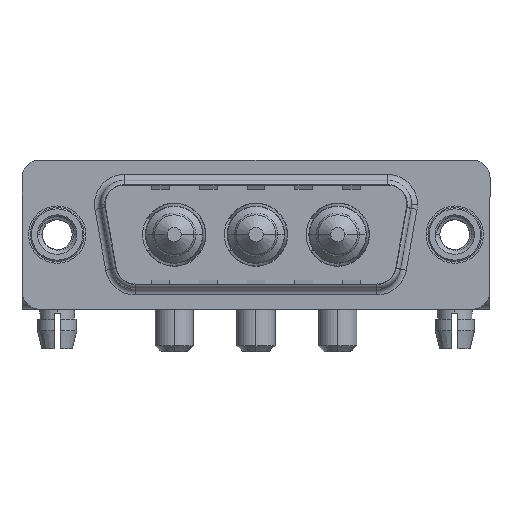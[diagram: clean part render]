
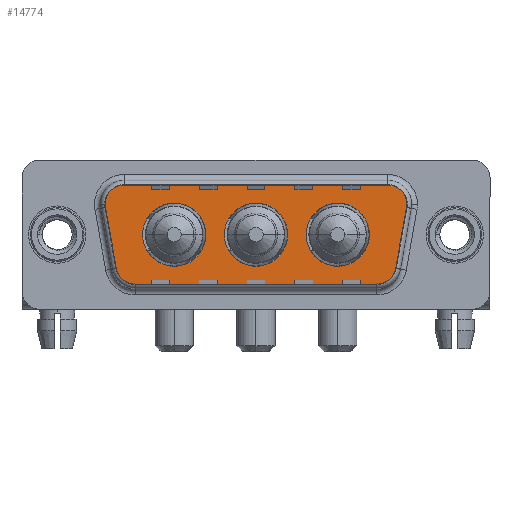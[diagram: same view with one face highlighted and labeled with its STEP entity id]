
A CAD part, top view. The second image highlights one B-rep face of the part: STEP entity #14774.
In plain terms, the highlighted planar face has unit normal (0, 0, 1).
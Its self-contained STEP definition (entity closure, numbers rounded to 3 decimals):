
#85 = AXIS2_PLACEMENT_3D ( 'NONE', #7280, #6156, #977 ) ;
#623 = DIRECTION ( 'NONE',  ( 0., 0., 1. ) ) ;
#839 = LINE ( 'NONE', #14089, #12455 ) ;
#970 = DIRECTION ( 'NONE',  ( 0., 0., 1. ) ) ;
#977 = DIRECTION ( 'NONE',  ( 1., 0., 0. ) ) ;
#1140 = CARTESIAN_POINT ( 'NONE',  ( 6.434, -4.9, 0. ) ) ;
#1514 = ORIENTED_EDGE ( 'NONE', *, *, #14882, .T. ) ;
#1573 = VERTEX_POINT ( 'NONE', #12220 ) ;
#1735 = CARTESIAN_POINT ( 'NONE',  ( 23.5, 0., 0. ) ) ;
#1796 = EDGE_CURVE ( 'NONE', #4521, #13586, #2761, .T. ) ;
#1833 = VERTEX_POINT ( 'NONE', #7849 ) ;
#2042 = DIRECTION ( 'NONE',  ( 0., 0., 1. ) ) ;
#2134 = DIRECTION ( 'NONE',  ( 0., 0., 1. ) ) ;
#2305 = CARTESIAN_POINT ( 'NONE',  ( 27.889, 4.9, 0. ) ) ;
#2618 = EDGE_CURVE ( 'NONE', #16424, #9800, #5568, .T. ) ;
#2658 = EDGE_CURVE ( 'NONE', #6936, #8131, #15450, .T. ) ;
#2761 = CIRCLE ( 'NONE', #7156, 2.65 ) ;
#3028 = DIRECTION ( 'NONE',  ( 0., 0., 1. ) ) ;
#3117 = VERTEX_POINT ( 'NONE', #4864 ) ;
#3252 = ORIENTED_EDGE ( 'NONE', *, *, #7204, .F. ) ;
#3288 = PLANE ( 'NONE',  #4502 ) ;
#3499 = DIRECTION ( 'NONE',  ( -1., 0., 0. ) ) ;
#3552 = AXIS2_PLACEMENT_3D ( 'NONE', #1735, #6993, #4160 ) ;
#3578 = EDGE_CURVE ( 'NONE', #7042, #1833, #839, .T. ) ;
#3691 = ORIENTED_EDGE ( 'NONE', *, *, #2618, .F. ) ;
#3872 = EDGE_LOOP ( 'NONE', ( #16402, #11729, #12885, #12441, #4454, #10476, #14609, #1514, #11324 ) ) ;
#3940 = ORIENTED_EDGE ( 'NONE', *, *, #1796, .F. ) ;
#3994 = AXIS2_PLACEMENT_3D ( 'NONE', #7100, #623, #4341 ) ;
#4160 = DIRECTION ( 'NONE',  ( 1., 0., 0. ) ) ;
#4191 = DIRECTION ( 'NONE',  ( 0., 0., 1. ) ) ;
#4214 = EDGE_CURVE ( 'NONE', #16069, #14965, #6508, .T. ) ;
#4341 = DIRECTION ( 'NONE',  ( 1., 0., 0. ) ) ;
#4454 = ORIENTED_EDGE ( 'NONE', *, *, #14383, .T. ) ;
#4468 = AXIS2_PLACEMENT_3D ( 'NONE', #15277, #2042, #3499 ) ;
#4502 = AXIS2_PLACEMENT_3D ( 'NONE', #6135, #11376, #7505 ) ;
#4521 = VERTEX_POINT ( 'NONE', #11869 ) ;
#4583 = ORIENTED_EDGE ( 'NONE', *, *, #13232, .F. ) ;
#4864 = CARTESIAN_POINT ( 'NONE',  ( 26.866, -4.9, 0. ) ) ;
#4932 = CARTESIAN_POINT ( 'NONE',  ( 6.434, -2.9, 0. ) ) ;
#4954 = CARTESIAN_POINT ( 'NONE',  ( 5.411, 4.9, 0. ) ) ;
#5054 = CARTESIAN_POINT ( 'NONE',  ( 29.889, 2.9, 0. ) ) ;
#5212 = DIRECTION ( 'NONE',  ( 0., 0., 1. ) ) ;
#5328 = VECTOR ( 'NONE', #10114, 1000. ) ;
#5332 = EDGE_CURVE ( 'NONE', #9641, #7042, #14146, .T. ) ;
#5568 = CIRCLE ( 'NONE', #6933, 2.65 ) ;
#5893 = AXIS2_PLACEMENT_3D ( 'NONE', #11986, #3028, #10776 ) ;
#6127 = DIRECTION ( 'NONE',  ( 0., 0., 1. ) ) ;
#6135 = CARTESIAN_POINT ( 'NONE',  ( 26.866, -2.9, 0. ) ) ;
#6156 = DIRECTION ( 'NONE',  ( 0., 0., 1. ) ) ;
#6275 = DIRECTION ( 'NONE',  ( 0.174, -0.985, 0. ) ) ;
#6508 = LINE ( 'NONE', #11746, #7497 ) ;
#6550 = DIRECTION ( 'NONE',  ( 1., 0., 0. ) ) ;
#6854 = VECTOR ( 'NONE', #7526, 1000. ) ;
#6855 = CARTESIAN_POINT ( 'NONE',  ( 28.836, -3.247, 0. ) ) ;
#6933 = AXIS2_PLACEMENT_3D ( 'NONE', #8158, #4191, #9444 ) ;
#6936 = VERTEX_POINT ( 'NONE', #5054 ) ;
#6993 = DIRECTION ( 'NONE',  ( 0., 0., 1. ) ) ;
#7033 = EDGE_CURVE ( 'NONE', #14965, #6936, #10509, .T. ) ;
#7042 = VERTEX_POINT ( 'NONE', #12782 ) ;
#7100 = CARTESIAN_POINT ( 'NONE',  ( 9.8, 0., 0. ) ) ;
#7156 = AXIS2_PLACEMENT_3D ( 'NONE', #7416, #6127, #6550 ) ;
#7166 = FACE_BOUND ( 'NONE', #11621, .T. ) ;
#7204 = EDGE_CURVE ( 'NONE', #9800, #16424, #10034, .T. ) ;
#7255 = DIRECTION ( 'NONE',  ( 0., 0., 1. ) ) ;
#7262 = AXIS2_PLACEMENT_3D ( 'NONE', #4932, #7255, #12490 ) ;
#7280 = CARTESIAN_POINT ( 'NONE',  ( 16.65, 0., 0. ) ) ;
#7416 = CARTESIAN_POINT ( 'NONE',  ( 16.65, 0., 0. ) ) ;
#7497 = VECTOR ( 'NONE', #15873, 1000. ) ;
#7505 = DIRECTION ( 'NONE',  ( 1., 0., 0. ) ) ;
#7526 = DIRECTION ( 'NONE',  ( 1., 0., 0. ) ) ;
#7819 = EDGE_LOOP ( 'NONE', ( #4583, #12108 ) ) ;
#7849 = CARTESIAN_POINT ( 'NONE',  ( 4.464, -3.247, 0. ) ) ;
#7879 = DIRECTION ( 'NONE',  ( 1., 0., 0. ) ) ;
#7903 = VERTEX_POINT ( 'NONE', #14605 ) ;
#8131 = VERTEX_POINT ( 'NONE', #2305 ) ;
#8158 = CARTESIAN_POINT ( 'NONE',  ( 9.8, 0., 0. ) ) ;
#8536 = EDGE_CURVE ( 'NONE', #13586, #4521, #14114, .T. ) ;
#8818 = LINE ( 'NONE', #14048, #6854 ) ;
#8842 = VERTEX_POINT ( 'NONE', #1140 ) ;
#8958 = EDGE_CURVE ( 'NONE', #1573, #7903, #16547, .T. ) ;
#9056 = CARTESIAN_POINT ( 'NONE',  ( 14., 0., 0. ) ) ;
#9444 = DIRECTION ( 'NONE',  ( 1., 0., 0. ) ) ;
#9641 = VERTEX_POINT ( 'NONE', #14588 ) ;
#9800 = VERTEX_POINT ( 'NONE', #13456 ) ;
#9999 = CIRCLE ( 'NONE', #14913, 2. ) ;
#10034 = CIRCLE ( 'NONE', #3994, 2.65 ) ;
#10114 = DIRECTION ( 'NONE',  ( -1., 0., 0. ) ) ;
#10476 = ORIENTED_EDGE ( 'NONE', *, *, #5332, .T. ) ;
#10509 = CIRCLE ( 'NONE', #11880, 2. ) ;
#10587 = ORIENTED_EDGE ( 'NONE', *, *, #8536, .F. ) ;
#10776 = DIRECTION ( 'NONE',  ( 1., 0., 0. ) ) ;
#11324 = ORIENTED_EDGE ( 'NONE', *, *, #12970, .T. ) ;
#11376 = DIRECTION ( 'NONE',  ( 0., 0., 1. ) ) ;
#11621 = EDGE_LOOP ( 'NONE', ( #3252, #3691 ) ) ;
#11680 = AXIS2_PLACEMENT_3D ( 'NONE', #16874, #970, #12917 ) ;
#11729 = ORIENTED_EDGE ( 'NONE', *, *, #4214, .T. ) ;
#11746 = CARTESIAN_POINT ( 'NONE',  ( 29.859, 2.553, 0. ) ) ;
#11869 = CARTESIAN_POINT ( 'NONE',  ( 19.3, 0., 0. ) ) ;
#11880 = AXIS2_PLACEMENT_3D ( 'NONE', #13903, #2134, #12689 ) ;
#11986 = CARTESIAN_POINT ( 'NONE',  ( 23.5, 0., 0. ) ) ;
#12060 = CIRCLE ( 'NONE', #3552, 2.65 ) ;
#12108 = ORIENTED_EDGE ( 'NONE', *, *, #8958, .F. ) ;
#12220 = CARTESIAN_POINT ( 'NONE',  ( 20.85, 0., 0. ) ) ;
#12441 = ORIENTED_EDGE ( 'NONE', *, *, #2658, .T. ) ;
#12455 = VECTOR ( 'NONE', #6275, 1000. ) ;
#12490 = DIRECTION ( 'NONE',  ( -1., 0., 0. ) ) ;
#12675 = CARTESIAN_POINT ( 'NONE',  ( 26.866, -2.9, 0. ) ) ;
#12689 = DIRECTION ( 'NONE',  ( -1., 0., 0. ) ) ;
#12743 = FACE_BOUND ( 'NONE', #15387, .T. ) ;
#12782 = CARTESIAN_POINT ( 'NONE',  ( 3.441, 2.553, 0. ) ) ;
#12885 = ORIENTED_EDGE ( 'NONE', *, *, #7033, .T. ) ;
#12917 = DIRECTION ( 'NONE',  ( 1., 0., 0. ) ) ;
#12970 = EDGE_CURVE ( 'NONE', #8842, #3117, #8818, .T. ) ;
#13232 = EDGE_CURVE ( 'NONE', #7903, #1573, #12060, .T. ) ;
#13456 = CARTESIAN_POINT ( 'NONE',  ( 12.45, 0., 0. ) ) ;
#13586 = VERTEX_POINT ( 'NONE', #9056 ) ;
#13903 = CARTESIAN_POINT ( 'NONE',  ( 27.889, 2.9, 0. ) ) ;
#14048 = CARTESIAN_POINT ( 'NONE',  ( 6.434, -4.9, 0. ) ) ;
#14089 = CARTESIAN_POINT ( 'NONE',  ( 3.441, 2.553, 0. ) ) ;
#14114 = CIRCLE ( 'NONE', #85, 2.65 ) ;
#14146 = CIRCLE ( 'NONE', #11680, 2. ) ;
#14383 = EDGE_CURVE ( 'NONE', #8131, #9641, #16634, .T. ) ;
#14407 = EDGE_CURVE ( 'NONE', #3117, #16069, #9999, .T. ) ;
#14588 = CARTESIAN_POINT ( 'NONE',  ( 5.411, 4.9, 0. ) ) ;
#14605 = CARTESIAN_POINT ( 'NONE',  ( 26.15, 0., 0. ) ) ;
#14609 = ORIENTED_EDGE ( 'NONE', *, *, #3578, .T. ) ;
#14662 = CIRCLE ( 'NONE', #7262, 2. ) ;
#14774 = ADVANCED_FACE ( 'NONE', ( #12743, #15152, #7166, #16355 ), #3288, .T. ) ;
#14882 = EDGE_CURVE ( 'NONE', #1833, #8842, #14662, .T. ) ;
#14913 = AXIS2_PLACEMENT_3D ( 'NONE', #12675, #5212, #7879 ) ;
#14965 = VERTEX_POINT ( 'NONE', #15582 ) ;
#15152 = FACE_BOUND ( 'NONE', #7819, .T. ) ;
#15277 = CARTESIAN_POINT ( 'NONE',  ( 27.889, 2.9, 0. ) ) ;
#15387 = EDGE_LOOP ( 'NONE', ( #3940, #10587 ) ) ;
#15450 = CIRCLE ( 'NONE', #4468, 2. ) ;
#15582 = CARTESIAN_POINT ( 'NONE',  ( 29.859, 2.553, 0. ) ) ;
#15691 = CARTESIAN_POINT ( 'NONE',  ( 7.15, 0., 0. ) ) ;
#15873 = DIRECTION ( 'NONE',  ( 0.174, 0.985, 0. ) ) ;
#16069 = VERTEX_POINT ( 'NONE', #6855 ) ;
#16355 = FACE_OUTER_BOUND ( 'NONE', #3872, .T. ) ;
#16402 = ORIENTED_EDGE ( 'NONE', *, *, #14407, .T. ) ;
#16424 = VERTEX_POINT ( 'NONE', #15691 ) ;
#16547 = CIRCLE ( 'NONE', #5893, 2.65 ) ;
#16634 = LINE ( 'NONE', #4954, #5328 ) ;
#16874 = CARTESIAN_POINT ( 'NONE',  ( 5.411, 2.9, 0. ) ) ;
